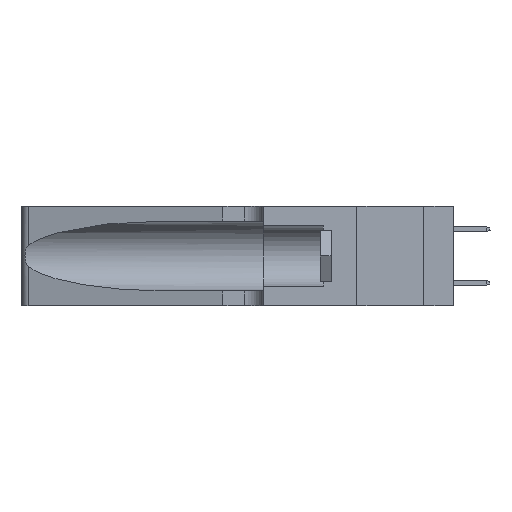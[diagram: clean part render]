
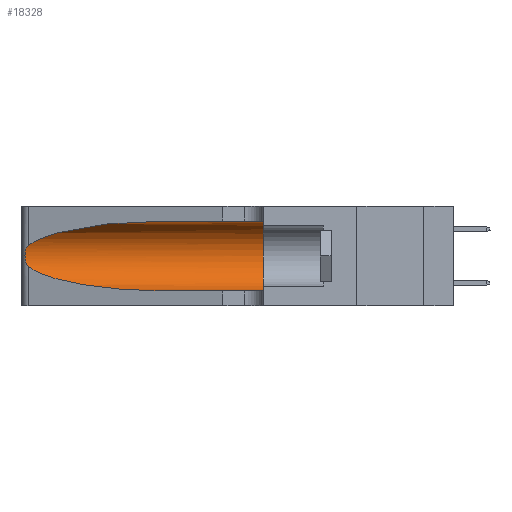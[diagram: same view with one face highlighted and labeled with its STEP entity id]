
A CAD part, left-side view. The second image highlights one B-rep face of the part: STEP entity #18328.
In plain terms, the highlighted cylindrical face has radius 3.308 mm (diameter 6.617 mm), a partial arc.
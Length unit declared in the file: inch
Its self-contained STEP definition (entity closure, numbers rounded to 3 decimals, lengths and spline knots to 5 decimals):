
#1949 = CARTESIAN_POINT ( 'NONE',  ( 0.26018, 1.23835, 0.19895 ) ) ;
#2146 = CARTESIAN_POINT ( 'NONE',  ( 0.25639, 1.23184, 0.21858 ) ) ;
#3117 = DIRECTION ( 'NONE',  ( 0., 0., -1. ) ) ;
#4004 = EDGE_CURVE ( 'NONE', #8036, #10112, #30050, .T. ) ;
#4928 = CARTESIAN_POINT ( 'NONE',  ( 0.2373, 1.15595, 0.28018 ) ) ;
#5045 = CARTESIAN_POINT ( 'NONE',  ( 0.25487, 1.22718, 0.22369 ) ) ;
#5225 = AXIS2_PLACEMENT_3D ( 'NONE', #13310, #32545, #9600 ) ;
#5262 = CARTESIAN_POINT ( 'NONE',  ( 0.25789, 1.23486, 0.15765 ) ) ;
#5377 = VERTEX_POINT ( 'NONE', #27477 ) ;
#5739 = VERTEX_POINT ( 'NONE', #10937 ) ;
#8036 = VERTEX_POINT ( 'NONE', #34354 ) ;
#8408 = CARTESIAN_POINT ( 'NONE',  ( 0.25856, 1.23593, 0.16098 ) ) ;
#9600 = DIRECTION ( 'NONE',  ( 0., 0., 1. ) ) ;
#9863 = CARTESIAN_POINT ( 'NONE',  ( 0.1305, 1.61858, 0.05475 ) ) ;
#10112 = VERTEX_POINT ( 'NONE', #31121 ) ;
#10283 =( BOUNDED_CURVE ( )  B_SPLINE_CURVE ( 3, ( #22615, #22808, #16957, #35563 ),
 .UNSPECIFIED., .F., .T. ) 
 B_SPLINE_CURVE_WITH_KNOTS ( ( 4, 4 ),
 ( 3.44316, 4.71239 ),
 .UNSPECIFIED. ) 
 CURVE ( )  GEOMETRIC_REPRESENTATION_ITEM ( )  RATIONAL_B_SPLINE_CURVE ( ( 1., 0.87, 0.87, 1. ) ) 
 REPRESENTATION_ITEM ( '' )  );
#10937 = CARTESIAN_POINT ( 'NONE',  ( 0.1305, 0.35, 0.05475 ) ) ;
#11649 = DIRECTION ( 'NONE',  ( 0., -1., 0. ) ) ;
#12484 = DIRECTION ( 'NONE',  ( 0., -1., 0. ) ) ;
#12686 = CYLINDRICAL_SURFACE ( 'NONE', #36929, 0.13025 ) ;
#13310 = CARTESIAN_POINT ( 'NONE',  ( 0.1305, 0.35, 0.185 ) ) ;
#13328 = ORIENTED_EDGE ( 'NONE', *, *, #40978, .T. ) ;
#14515 = CARTESIAN_POINT ( 'NONE',  ( 0.25487, 1.22718, 0.22369 ) ) ;
#14629 = CARTESIAN_POINT ( 'NONE',  ( 0.26075, 1.23896, 0.19203 ) ) ;
#15404 = LINE ( 'NONE', #31090, #16701 ) ;
#15533 = EDGE_CURVE ( 'NONE', #5377, #5739, #29270, .T. ) ;
#16701 = VECTOR ( 'NONE', #11649, 39.37008 ) ;
#16957 = CARTESIAN_POINT ( 'NONE',  ( 0.18966, 0.96281, 0.05475 ) ) ;
#17775 = CARTESIAN_POINT ( 'NONE',  ( 0.25555, 1.22994, 0.2215 ) ) ;
#17993 = CARTESIAN_POINT ( 'NONE',  ( 0.25639, 1.23186, 0.15144 ) ) ;
#18328 = ADVANCED_FACE ( 'NONE', ( #28582 ), #12686, .F. ) ;
#19976 = ORIENTED_EDGE ( 'NONE', *, *, #24903, .T. ) ;
#21126 = CARTESIAN_POINT ( 'NONE',  ( 0.25787, 1.23484, 0.2124 ) ) ;
#21242 = CIRCLE ( 'NONE', #5225, 0.13025 ) ;
#21331 = CARTESIAN_POINT ( 'NONE',  ( 0.25487, 1.22718, 0.14631 ) ) ;
#22118 = VERTEX_POINT ( 'NONE', #32556 ) ;
#22496 = EDGE_LOOP ( 'NONE', ( #28435, #19976, #13328, #33303, #35456, #23033 ) ) ;
#22615 = CARTESIAN_POINT ( 'NONE',  ( 0.25487, 1.22718, 0.14631 ) ) ;
#22808 = CARTESIAN_POINT ( 'NONE',  ( 0.2373, 1.15595, 0.08982 ) ) ;
#23033 = ORIENTED_EDGE ( 'NONE', *, *, #39873, .F. ) ;
#24450 = CARTESIAN_POINT ( 'NONE',  ( 0.26075, 1.23896, 0.178 ) ) ;
#24903 = EDGE_CURVE ( 'NONE', #10112, #22118, #39867, .T. ) ;
#27477 = CARTESIAN_POINT ( 'NONE',  ( 0.1305, 0.72297, 0.05475 ) ) ;
#27585 = CARTESIAN_POINT ( 'NONE',  ( 0.25555, 1.22993, 0.14849 ) ) ;
#28435 = ORIENTED_EDGE ( 'NONE', *, *, #4004, .T. ) ;
#28582 = FACE_OUTER_BOUND ( 'NONE', #22496, .T. ) ;
#29270 = LINE ( 'NONE', #9863, #32207 ) ;
#30050 =( BOUNDED_CURVE ( )  B_SPLINE_CURVE ( 3, ( #36693, #33551, #4928, #14515 ),
 .UNSPECIFIED., .F., .T. ) 
 B_SPLINE_CURVE_WITH_KNOTS ( ( 4, 4 ),
 ( 1.5708, 2.84003 ),
 .UNSPECIFIED. ) 
 CURVE ( )  GEOMETRIC_REPRESENTATION_ITEM ( )  RATIONAL_B_SPLINE_CURVE ( ( 1., 0.87, 0.87, 1. ) ) 
 REPRESENTATION_ITEM ( '' )  );
#30522 = CARTESIAN_POINT ( 'NONE',  ( 0.25854, 1.2359, 0.20912 ) ) ;
#30874 = VERTEX_POINT ( 'NONE', #31423 ) ;
#31090 = CARTESIAN_POINT ( 'NONE',  ( 0.1305, 1.61858, 0.31525 ) ) ;
#31121 = CARTESIAN_POINT ( 'NONE',  ( 0.25487, 1.22718, 0.22369 ) ) ;
#31423 = CARTESIAN_POINT ( 'NONE',  ( 0.1305, 0.35, 0.31525 ) ) ;
#32207 = VECTOR ( 'NONE', #35338, 39.37008 ) ;
#32545 = DIRECTION ( 'NONE',  ( 0., 1., 0. ) ) ;
#32556 = CARTESIAN_POINT ( 'NONE',  ( 0.25487, 1.22718, 0.14631 ) ) ;
#33303 = ORIENTED_EDGE ( 'NONE', *, *, #15533, .T. ) ;
#33551 = CARTESIAN_POINT ( 'NONE',  ( 0.18966, 0.96281, 0.31525 ) ) ;
#34354 = CARTESIAN_POINT ( 'NONE',  ( 0.1305, 0.72297, 0.31525 ) ) ;
#35338 = DIRECTION ( 'NONE',  ( 0., -1., 0. ) ) ;
#35456 = ORIENTED_EDGE ( 'NONE', *, *, #37214, .F. ) ;
#35563 = CARTESIAN_POINT ( 'NONE',  ( 0.1305, 0.72297, 0.05475 ) ) ;
#36693 = CARTESIAN_POINT ( 'NONE',  ( 0.1305, 0.72297, 0.31525 ) ) ;
#36929 = AXIS2_PLACEMENT_3D ( 'NONE', #41107, #12484, #3117 ) ;
#37006 = CARTESIAN_POINT ( 'NONE',  ( 0.26017, 1.23833, 0.17102 ) ) ;
#37214 = EDGE_CURVE ( 'NONE', #30874, #5739, #21242, .T. ) ;
#39867 = B_SPLINE_CURVE_WITH_KNOTS ( 'NONE', 3,
 ( #5045, #17775, #2146, #21126, #30522, #1949, #14629, #24450, #37006, #8408, #5262, #17993, #27585, #21331 ),
 .UNSPECIFIED., .F., .F.,
 ( 4, 2, 2, 2, 2, 2, 4 ),
 ( 0., 0.00027, 0.00053, 0.00107, 0.0016, 0.00187, 0.00214 ),
 .UNSPECIFIED. ) ;
#39873 = EDGE_CURVE ( 'NONE', #8036, #30874, #15404, .T. ) ;
#40978 = EDGE_CURVE ( 'NONE', #22118, #5377, #10283, .T. ) ;
#41107 = CARTESIAN_POINT ( 'NONE',  ( 0.1305, 1.61858, 0.185 ) ) ;
